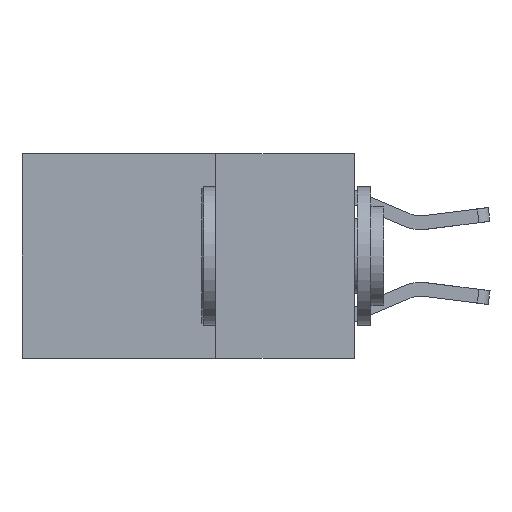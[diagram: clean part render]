
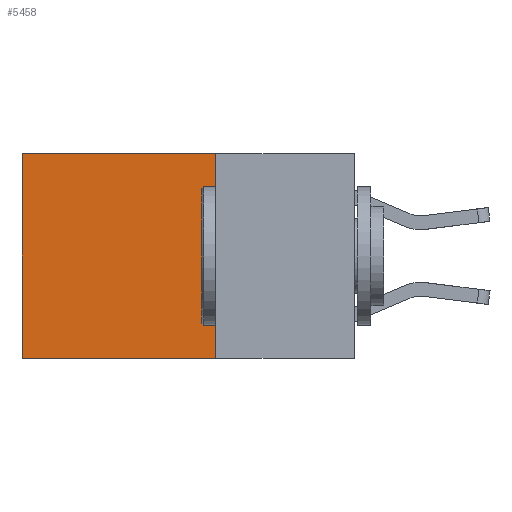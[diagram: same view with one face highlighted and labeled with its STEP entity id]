
A CAD part, left-side view. The second image highlights one B-rep face of the part: STEP entity #5458.
In plain terms, the highlighted planar face has unit normal (-1, 0, 0).
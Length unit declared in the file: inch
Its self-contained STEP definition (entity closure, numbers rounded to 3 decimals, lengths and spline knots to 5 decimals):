
#25 = EDGE_CURVE ( 'NONE', #12167, #10726, #7879, .T. ) ;
#56 = DIRECTION ( 'NONE',  ( 0., 1., 0. ) ) ;
#352 = LINE ( 'NONE', #9035, #7610 ) ;
#760 = CARTESIAN_POINT ( 'NONE',  ( 0.2625, 0.25, 0. ) ) ;
#791 = ORIENTED_EDGE ( 'NONE', *, *, #12524, .T. ) ;
#1330 = VECTOR ( 'NONE', #56, 39.37008 ) ;
#1339 = AXIS2_PLACEMENT_3D ( 'NONE', #760, #9643, #6613 ) ;
#1946 = CARTESIAN_POINT ( 'NONE',  ( 0.2625, 0.6, -0.37 ) ) ;
#2163 = DIRECTION ( 'NONE',  ( 0., 1., 0. ) ) ;
#2330 = VECTOR ( 'NONE', #6912, 39.37008 ) ;
#2506 = CARTESIAN_POINT ( 'NONE',  ( 0.2625, 0.6, 0. ) ) ;
#2937 = CARTESIAN_POINT ( 'NONE',  ( 0.2625, 0.25, 0. ) ) ;
#3914 = EDGE_LOOP ( 'NONE', ( #5721, #7120, #12393, #791 ) ) ;
#3918 = CARTESIAN_POINT ( 'NONE',  ( 0.2625, 0.25, 0. ) ) ;
#4602 = VERTEX_POINT ( 'NONE', #1946 ) ;
#4930 = CARTESIAN_POINT ( 'NONE',  ( 0.2625, 0.25, -0.37 ) ) ;
#5089 = EDGE_CURVE ( 'NONE', #10726, #4602, #11867, .T. ) ;
#5458 = ADVANCED_FACE ( 'NONE', ( #11006 ), #6060, .F. ) ;
#5721 = ORIENTED_EDGE ( 'NONE', *, *, #10814, .T. ) ;
#6060 = PLANE ( 'NONE',  #1339 ) ;
#6613 = DIRECTION ( 'NONE',  ( 0., 0., -1. ) ) ;
#6912 = DIRECTION ( 'NONE',  ( 0., 0., -1. ) ) ;
#7120 = ORIENTED_EDGE ( 'NONE', *, *, #5089, .F. ) ;
#7610 = VECTOR ( 'NONE', #2163, 39.37008 ) ;
#7804 = DIRECTION ( 'NONE',  ( 0., 0., -1. ) ) ;
#7879 = LINE ( 'NONE', #3918, #12766 ) ;
#8137 = CARTESIAN_POINT ( 'NONE',  ( 0.2625, 0.6, 0. ) ) ;
#9035 = CARTESIAN_POINT ( 'NONE',  ( 0.2625, 0.25, 0. ) ) ;
#9643 = DIRECTION ( 'NONE',  ( 1., 0., 0. ) ) ;
#9937 = VERTEX_POINT ( 'NONE', #2506 ) ;
#10683 = CARTESIAN_POINT ( 'NONE',  ( 0.2625, 0.25, -0.37 ) ) ;
#10726 = VERTEX_POINT ( 'NONE', #10683 ) ;
#10814 = EDGE_CURVE ( 'NONE', #9937, #4602, #11926, .T. ) ;
#11006 = FACE_OUTER_BOUND ( 'NONE', #3914, .T. ) ;
#11867 = LINE ( 'NONE', #4930, #1330 ) ;
#11926 = LINE ( 'NONE', #8137, #2330 ) ;
#12167 = VERTEX_POINT ( 'NONE', #2937 ) ;
#12393 = ORIENTED_EDGE ( 'NONE', *, *, #25, .F. ) ;
#12524 = EDGE_CURVE ( 'NONE', #12167, #9937, #352, .T. ) ;
#12766 = VECTOR ( 'NONE', #7804, 39.37008 ) ;
